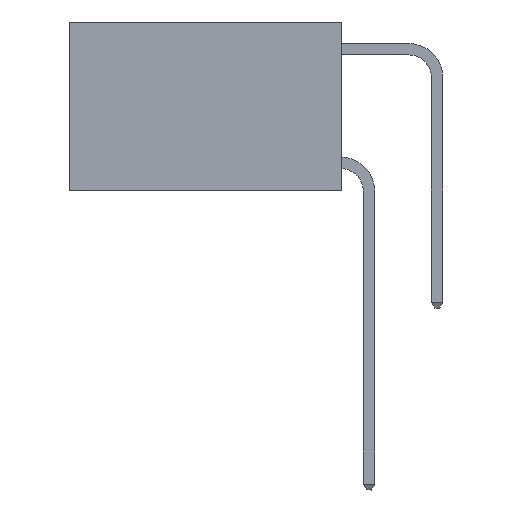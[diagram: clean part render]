
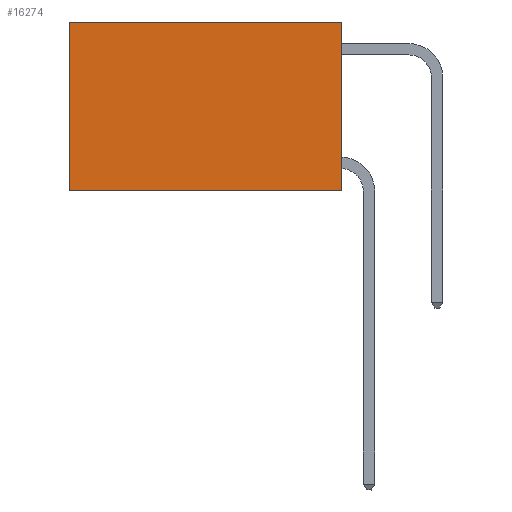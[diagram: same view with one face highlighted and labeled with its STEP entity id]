
A CAD part, left-side view. The second image highlights one B-rep face of the part: STEP entity #16274.
In plain terms, the highlighted planar face has unit normal (-1, 0, 0).
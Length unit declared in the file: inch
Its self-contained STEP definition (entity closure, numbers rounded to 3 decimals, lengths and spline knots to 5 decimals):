
#64 = VECTOR ( 'NONE', #3068, 39.37008 ) ;
#877 = VECTOR ( 'NONE', #4682, 39.37008 ) ;
#984 = ORIENTED_EDGE ( 'NONE', *, *, #10738, .T. ) ;
#1019 = ORIENTED_EDGE ( 'NONE', *, *, #3689, .F. ) ;
#1799 = CARTESIAN_POINT ( 'NONE',  ( 0.2625, 0., 0. ) ) ;
#2072 = EDGE_CURVE ( 'NONE', #8091, #8265, #15053, .T. ) ;
#2125 = ORIENTED_EDGE ( 'NONE', *, *, #2072, .T. ) ;
#3068 = DIRECTION ( 'NONE',  ( 0., 0., -1. ) ) ;
#3471 = DIRECTION ( 'NONE',  ( 1., 0., 0. ) ) ;
#3689 = EDGE_CURVE ( 'NONE', #8091, #14186, #4478, .T. ) ;
#4267 = AXIS2_PLACEMENT_3D ( 'NONE', #1799, #3471, #14915 ) ;
#4478 = LINE ( 'NONE', #7982, #64 ) ;
#4682 = DIRECTION ( 'NONE',  ( 0., 1., 0. ) ) ;
#5347 = VECTOR ( 'NONE', #15507, 39.37008 ) ;
#5969 = DIRECTION ( 'NONE',  ( 0., 0., -1. ) ) ;
#7765 = CARTESIAN_POINT ( 'NONE',  ( 0.2625, 0.6, -0.37 ) ) ;
#7982 = CARTESIAN_POINT ( 'NONE',  ( 0.2625, 0., 0. ) ) ;
#8091 = VERTEX_POINT ( 'NONE', #14818 ) ;
#8228 = ORIENTED_EDGE ( 'NONE', *, *, #15574, .F. ) ;
#8265 = VERTEX_POINT ( 'NONE', #18462 ) ;
#9947 = FACE_OUTER_BOUND ( 'NONE', #14689, .T. ) ;
#10738 = EDGE_CURVE ( 'NONE', #8265, #19575, #19318, .T. ) ;
#11204 = CARTESIAN_POINT ( 'NONE',  ( 0.2625, 0., -0.37 ) ) ;
#11683 = PLANE ( 'NONE',  #4267 ) ;
#11730 = CARTESIAN_POINT ( 'NONE',  ( 0.2625, 0., 0. ) ) ;
#12501 = CARTESIAN_POINT ( 'NONE',  ( 0.2625, 0.6, 0. ) ) ;
#14186 = VERTEX_POINT ( 'NONE', #11204 ) ;
#14689 = EDGE_LOOP ( 'NONE', ( #984, #8228, #1019, #2125 ) ) ;
#14818 = CARTESIAN_POINT ( 'NONE',  ( 0.2625, 0., 0. ) ) ;
#14915 = DIRECTION ( 'NONE',  ( 0., 0., -1. ) ) ;
#15045 = VECTOR ( 'NONE', #5969, 39.37008 ) ;
#15053 = LINE ( 'NONE', #11730, #5347 ) ;
#15507 = DIRECTION ( 'NONE',  ( 0., 1., 0. ) ) ;
#15574 = EDGE_CURVE ( 'NONE', #14186, #19575, #18280, .T. ) ;
#16274 = ADVANCED_FACE ( 'NONE', ( #9947 ), #11683, .F. ) ;
#17703 = CARTESIAN_POINT ( 'NONE',  ( 0.2625, 0., -0.37 ) ) ;
#18280 = LINE ( 'NONE', #17703, #877 ) ;
#18462 = CARTESIAN_POINT ( 'NONE',  ( 0.2625, 0.6, 0. ) ) ;
#19318 = LINE ( 'NONE', #12501, #15045 ) ;
#19575 = VERTEX_POINT ( 'NONE', #7765 ) ;
